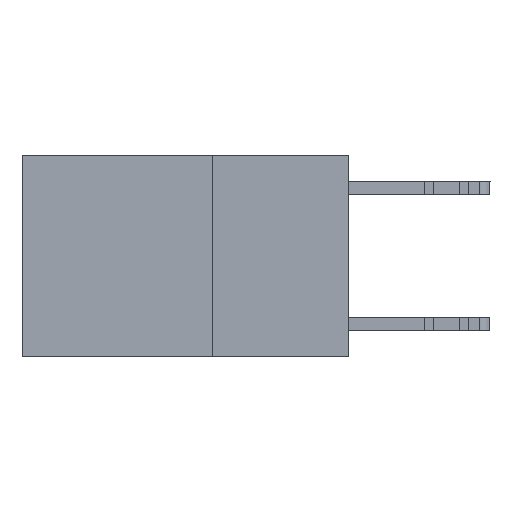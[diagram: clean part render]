
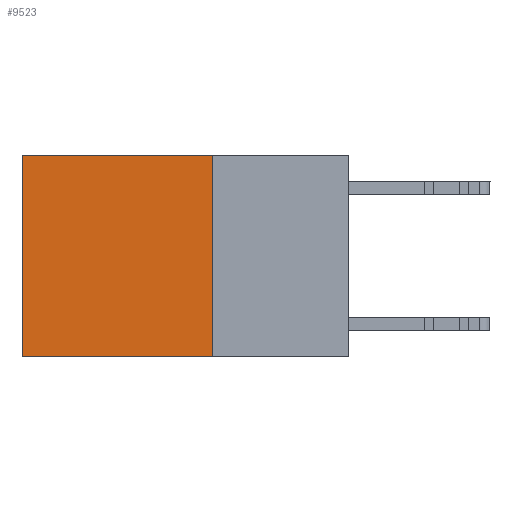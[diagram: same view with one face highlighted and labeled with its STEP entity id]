
A CAD part, left-side view. The second image highlights one B-rep face of the part: STEP entity #9523.
In plain terms, the highlighted planar face has unit normal (-1, 0, 0).
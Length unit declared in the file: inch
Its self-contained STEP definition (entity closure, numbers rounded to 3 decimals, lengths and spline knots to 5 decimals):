
#543 = VERTEX_POINT ( 'NONE', #17014 ) ;
#2958 = FACE_OUTER_BOUND ( 'NONE', #6255, .T. ) ;
#4221 = ORIENTED_EDGE ( 'NONE', *, *, #24521, .F. ) ;
#6183 = CARTESIAN_POINT ( 'NONE',  ( 0.2625, 0.25, 0. ) ) ;
#6255 = EDGE_LOOP ( 'NONE', ( #7880, #7519, #4221, #6921 ) ) ;
#6921 = ORIENTED_EDGE ( 'NONE', *, *, #29665, .T. ) ;
#7519 = ORIENTED_EDGE ( 'NONE', *, *, #19379, .F. ) ;
#7880 = ORIENTED_EDGE ( 'NONE', *, *, #18059, .T. ) ;
#9256 = VECTOR ( 'NONE', #27723, 39.37008 ) ;
#9523 = ADVANCED_FACE ( 'NONE', ( #2958 ), #25045, .F. ) ;
#10221 = DIRECTION ( 'NONE',  ( 1., 0., 0. ) ) ;
#11541 = DIRECTION ( 'NONE',  ( 0., 0., -1. ) ) ;
#11702 = VECTOR ( 'NONE', #30841, 39.37008 ) ;
#12234 = VECTOR ( 'NONE', #20135, 39.37008 ) ;
#12575 = CARTESIAN_POINT ( 'NONE',  ( 0.2625, 0.25, 0. ) ) ;
#12698 = CARTESIAN_POINT ( 'NONE',  ( 0.2625, 0.25, -0.37 ) ) ;
#13124 = VERTEX_POINT ( 'NONE', #29769 ) ;
#15084 = LINE ( 'NONE', #19982, #12234 ) ;
#15974 = VERTEX_POINT ( 'NONE', #12698 ) ;
#16797 = LINE ( 'NONE', #30998, #11702 ) ;
#17014 = CARTESIAN_POINT ( 'NONE',  ( 0.2625, 0.6, 0. ) ) ;
#17472 = DIRECTION ( 'NONE',  ( 0., 0., -1. ) ) ;
#17593 = VECTOR ( 'NONE', #11541, 39.37008 ) ;
#17728 = LINE ( 'NONE', #25762, #17593 ) ;
#18059 = EDGE_CURVE ( 'NONE', #543, #13124, #15084, .T. ) ;
#19379 = EDGE_CURVE ( 'NONE', #15974, #13124, #19843, .T. ) ;
#19843 = LINE ( 'NONE', #29467, #9256 ) ;
#19982 = CARTESIAN_POINT ( 'NONE',  ( 0.2625, 0.6, 0. ) ) ;
#20135 = DIRECTION ( 'NONE',  ( 0., 0., -1. ) ) ;
#20388 = VERTEX_POINT ( 'NONE', #6183 ) ;
#21522 = AXIS2_PLACEMENT_3D ( 'NONE', #12575, #10221, #17472 ) ;
#24521 = EDGE_CURVE ( 'NONE', #20388, #15974, #17728, .T. ) ;
#25045 = PLANE ( 'NONE',  #21522 ) ;
#25762 = CARTESIAN_POINT ( 'NONE',  ( 0.2625, 0.25, 0. ) ) ;
#27723 = DIRECTION ( 'NONE',  ( 0., 1., 0. ) ) ;
#29467 = CARTESIAN_POINT ( 'NONE',  ( 0.2625, 0.25, -0.37 ) ) ;
#29665 = EDGE_CURVE ( 'NONE', #20388, #543, #16797, .T. ) ;
#29769 = CARTESIAN_POINT ( 'NONE',  ( 0.2625, 0.6, -0.37 ) ) ;
#30841 = DIRECTION ( 'NONE',  ( 0., 1., 0. ) ) ;
#30998 = CARTESIAN_POINT ( 'NONE',  ( 0.2625, 0.25, 0. ) ) ;
